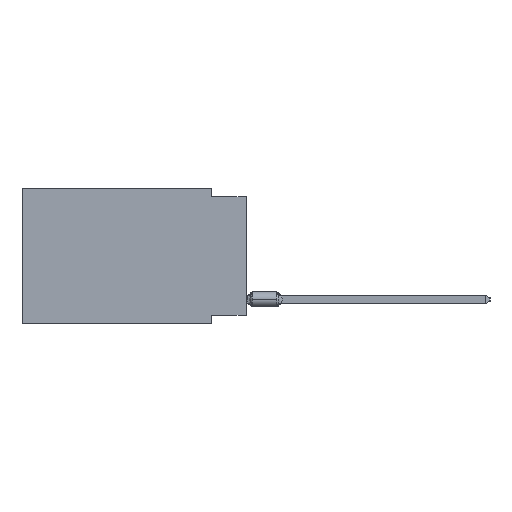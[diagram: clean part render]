
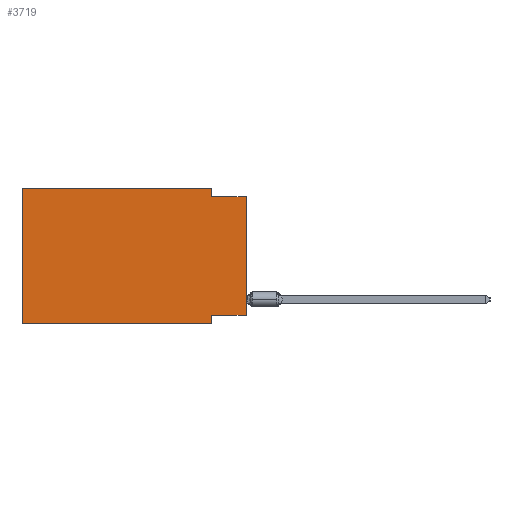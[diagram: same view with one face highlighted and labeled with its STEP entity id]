
A CAD part, left-side view. The second image highlights one B-rep face of the part: STEP entity #3719.
In plain terms, the highlighted planar face has unit normal (-1, 0, 0).
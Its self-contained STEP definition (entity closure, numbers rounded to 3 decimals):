
#1229 = VECTOR ( 'NONE', #30348, 1000. ) ;
#1543 = VECTOR ( 'NONE', #4166, 1000. ) ;
#3719 = ADVANCED_FACE ( 'NONE', ( #41553 ), #32791, .F. ) ;
#4166 = DIRECTION ( 'NONE',  ( 0., 1., 0. ) ) ;
#4559 = CARTESIAN_POINT ( 'NONE',  ( 0., 16.383, -9.906 ) ) ;
#5020 = DIRECTION ( 'NONE',  ( 0., 0., -1. ) ) ;
#5179 = CARTESIAN_POINT ( 'NONE',  ( 0., 16.383, 0. ) ) ;
#9013 = VERTEX_POINT ( 'NONE', #50935 ) ;
#9014 = LINE ( 'NONE', #41665, #46206 ) ;
#10107 = EDGE_CURVE ( 'NONE', #43273, #29289, #9014, .T. ) ;
#10755 = VERTEX_POINT ( 'NONE', #36712 ) ;
#11046 = LINE ( 'NONE', #44228, #30395 ) ;
#11806 = EDGE_CURVE ( 'NONE', #19458, #9013, #33366, .T. ) ;
#12061 = VERTEX_POINT ( 'NONE', #27755 ) ;
#13309 = EDGE_CURVE ( 'NONE', #19458, #12061, #11046, .T. ) ;
#14064 = VERTEX_POINT ( 'NONE', #24293 ) ;
#14148 = CARTESIAN_POINT ( 'NONE',  ( 0., 2.54, -9.906 ) ) ;
#14833 = ORIENTED_EDGE ( 'NONE', *, *, #10107, .F. ) ;
#17045 = EDGE_CURVE ( 'NONE', #44052, #10755, #40425, .T. ) ;
#17300 = AXIS2_PLACEMENT_3D ( 'NONE', #5179, #40765, #20587 ) ;
#17425 = VECTOR ( 'NONE', #45398, 1000. ) ;
#17517 = ORIENTED_EDGE ( 'NONE', *, *, #17045, .T. ) ;
#18189 = LINE ( 'NONE', #42628, #40785 ) ;
#19458 = VERTEX_POINT ( 'NONE', #26757 ) ;
#20489 = ORIENTED_EDGE ( 'NONE', *, *, #11806, .F. ) ;
#20587 = DIRECTION ( 'NONE',  ( 0., 0., -1. ) ) ;
#21251 = ORIENTED_EDGE ( 'NONE', *, *, #41127, .F. ) ;
#21340 = LINE ( 'NONE', #37283, #36799 ) ;
#24293 = CARTESIAN_POINT ( 'NONE',  ( 0., 16.383, 0. ) ) ;
#26228 = CARTESIAN_POINT ( 'NONE',  ( 0., 16.383, -9.906 ) ) ;
#26757 = CARTESIAN_POINT ( 'NONE',  ( 0., 0., -9.271 ) ) ;
#27755 = CARTESIAN_POINT ( 'NONE',  ( 0., 0., -0.635 ) ) ;
#29289 = VERTEX_POINT ( 'NONE', #32674 ) ;
#30348 = DIRECTION ( 'NONE',  ( 0., 0., -1. ) ) ;
#30395 = VECTOR ( 'NONE', #40243, 1000. ) ;
#31370 = EDGE_CURVE ( 'NONE', #29289, #12061, #21340, .T. ) ;
#32674 = CARTESIAN_POINT ( 'NONE',  ( 0., 2.54, -0.635 ) ) ;
#32791 = PLANE ( 'NONE',  #17300 ) ;
#33366 = LINE ( 'NONE', #49297, #1543 ) ;
#34087 = ORIENTED_EDGE ( 'NONE', *, *, #31370, .F. ) ;
#34641 = EDGE_LOOP ( 'NONE', ( #36085, #34087, #14833, #40501, #21251, #17517, #35861, #20489 ) ) ;
#35861 = ORIENTED_EDGE ( 'NONE', *, *, #46889, .F. ) ;
#36085 = ORIENTED_EDGE ( 'NONE', *, *, #13309, .T. ) ;
#36712 = CARTESIAN_POINT ( 'NONE',  ( 0., 2.54, -9.906 ) ) ;
#36799 = VECTOR ( 'NONE', #45773, 1000. ) ;
#37283 = CARTESIAN_POINT ( 'NONE',  ( 0., 0., -0.635 ) ) ;
#37498 = DIRECTION ( 'NONE',  ( 0., -1., 0. ) ) ;
#38862 = VECTOR ( 'NONE', #37498, 1000. ) ;
#40243 = DIRECTION ( 'NONE',  ( 0., 0., 1. ) ) ;
#40425 = LINE ( 'NONE', #4559, #38862 ) ;
#40501 = ORIENTED_EDGE ( 'NONE', *, *, #45197, .F. ) ;
#40765 = DIRECTION ( 'NONE',  ( 1., 0., 0. ) ) ;
#40785 = VECTOR ( 'NONE', #51098, 1000. ) ;
#41127 = EDGE_CURVE ( 'NONE', #44052, #14064, #50153, .T. ) ;
#41553 = FACE_OUTER_BOUND ( 'NONE', #34641, .T. ) ;
#41665 = CARTESIAN_POINT ( 'NONE',  ( 0., 2.54, 0. ) ) ;
#41674 = CARTESIAN_POINT ( 'NONE',  ( 0., 16.383, 0. ) ) ;
#42628 = CARTESIAN_POINT ( 'NONE',  ( 0., 16.383, 0. ) ) ;
#43273 = VERTEX_POINT ( 'NONE', #47041 ) ;
#44052 = VERTEX_POINT ( 'NONE', #26228 ) ;
#44228 = CARTESIAN_POINT ( 'NONE',  ( 0., 0., 0. ) ) ;
#45197 = EDGE_CURVE ( 'NONE', #14064, #43273, #18189, .T. ) ;
#45398 = DIRECTION ( 'NONE',  ( 0., 0., 1. ) ) ;
#45773 = DIRECTION ( 'NONE',  ( 0., -1., 0. ) ) ;
#46206 = VECTOR ( 'NONE', #5020, 1000. ) ;
#46889 = EDGE_CURVE ( 'NONE', #9013, #10755, #50518, .T. ) ;
#47041 = CARTESIAN_POINT ( 'NONE',  ( 0., 2.54, 0. ) ) ;
#49297 = CARTESIAN_POINT ( 'NONE',  ( 0., 0., -9.271 ) ) ;
#50153 = LINE ( 'NONE', #41674, #17425 ) ;
#50518 = LINE ( 'NONE', #14148, #1229 ) ;
#50935 = CARTESIAN_POINT ( 'NONE',  ( 0., 2.54, -9.271 ) ) ;
#51098 = DIRECTION ( 'NONE',  ( 0., -1., 0. ) ) ;
